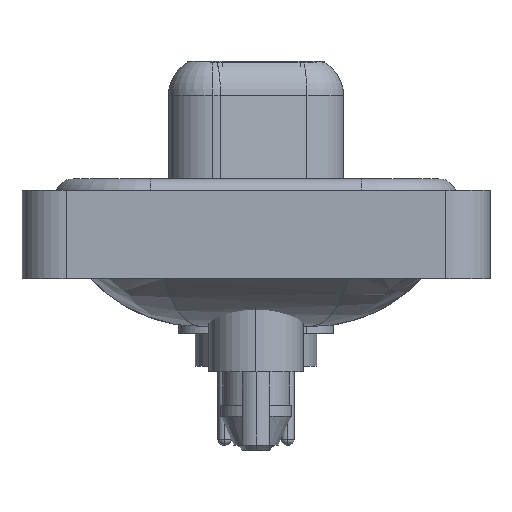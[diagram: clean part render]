
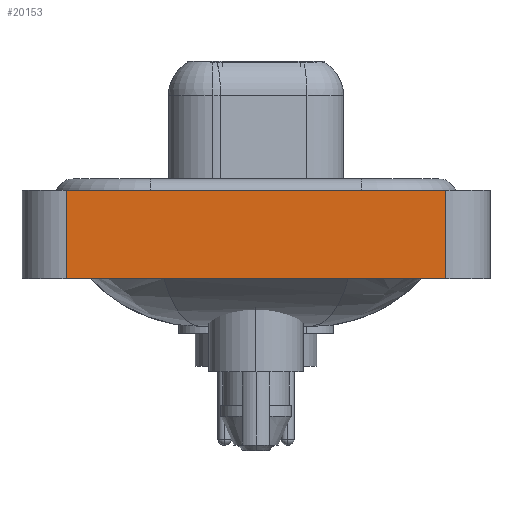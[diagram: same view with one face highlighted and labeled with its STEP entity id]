
A CAD part, left-side view. The second image highlights one B-rep face of the part: STEP entity #20153.
In plain terms, the highlighted planar face has unit normal (-1, 0, 0).
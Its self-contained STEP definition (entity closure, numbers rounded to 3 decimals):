
#46 = CARTESIAN_POINT ( 'NONE',  ( -7.35, -8.55, -3.6 ) ) ;
#87 = DIRECTION ( 'NONE',  ( 0., -1., 0. ) ) ;
#1647 = EDGE_CURVE ( 'NONE', #10196, #20357, #12779, .T. ) ;
#2560 = AXIS2_PLACEMENT_3D ( 'NONE', #13765, #23207, #22956 ) ;
#5032 = LINE ( 'NONE', #21551, #9529 ) ;
#5711 = ORIENTED_EDGE ( 'NONE', *, *, #6434, .F. ) ;
#5969 = LINE ( 'NONE', #19021, #17389 ) ;
#6434 = EDGE_CURVE ( 'NONE', #22439, #9932, #5969, .T. ) ;
#6819 = DIRECTION ( 'NONE',  ( 0., -1., 0. ) ) ;
#7361 = LINE ( 'NONE', #16152, #7909 ) ;
#7904 = ORIENTED_EDGE ( 'NONE', *, *, #12205, .F. ) ;
#7909 = VECTOR ( 'NONE', #20059, 1000. ) ;
#8629 = CARTESIAN_POINT ( 'NONE',  ( -7.35, -8.55, -3.6 ) ) ;
#8754 = CARTESIAN_POINT ( 'NONE',  ( -7.35, -8.55, 0.4 ) ) ;
#9529 = VECTOR ( 'NONE', #15808, 1000. ) ;
#9932 = VERTEX_POINT ( 'NONE', #8754 ) ;
#10108 = FACE_OUTER_BOUND ( 'NONE', #12371, .T. ) ;
#10196 = VERTEX_POINT ( 'NONE', #21577 ) ;
#11215 = ORIENTED_EDGE ( 'NONE', *, *, #13314, .T. ) ;
#12205 = EDGE_CURVE ( 'NONE', #10196, #22439, #7361, .T. ) ;
#12371 = EDGE_LOOP ( 'NONE', ( #11215, #5711, #7904, #21185 ) ) ;
#12779 = LINE ( 'NONE', #8629, #19382 ) ;
#13314 = EDGE_CURVE ( 'NONE', #20357, #9932, #5032, .T. ) ;
#13765 = CARTESIAN_POINT ( 'NONE',  ( -7.35, -8.55, -3.6 ) ) ;
#15485 = PLANE ( 'NONE',  #2560 ) ;
#15808 = DIRECTION ( 'NONE',  ( 0., 0., 1. ) ) ;
#16152 = CARTESIAN_POINT ( 'NONE',  ( -7.35, 8.55, -3.6 ) ) ;
#17389 = VECTOR ( 'NONE', #87, 1000. ) ;
#19021 = CARTESIAN_POINT ( 'NONE',  ( -7.35, -8.55, 0.4 ) ) ;
#19382 = VECTOR ( 'NONE', #6819, 1000. ) ;
#20059 = DIRECTION ( 'NONE',  ( 0., 0., 1. ) ) ;
#20153 = ADVANCED_FACE ( 'NONE', ( #10108 ), #15485, .T. ) ;
#20357 = VERTEX_POINT ( 'NONE', #46 ) ;
#21185 = ORIENTED_EDGE ( 'NONE', *, *, #1647, .T. ) ;
#21261 = CARTESIAN_POINT ( 'NONE',  ( -7.35, 8.55, 0.4 ) ) ;
#21551 = CARTESIAN_POINT ( 'NONE',  ( -7.35, -8.55, -3.6 ) ) ;
#21577 = CARTESIAN_POINT ( 'NONE',  ( -7.35, 8.55, -3.6 ) ) ;
#22439 = VERTEX_POINT ( 'NONE', #21261 ) ;
#22956 = DIRECTION ( 'NONE',  ( 0., 0., 1. ) ) ;
#23207 = DIRECTION ( 'NONE',  ( -1., 0., 0. ) ) ;
